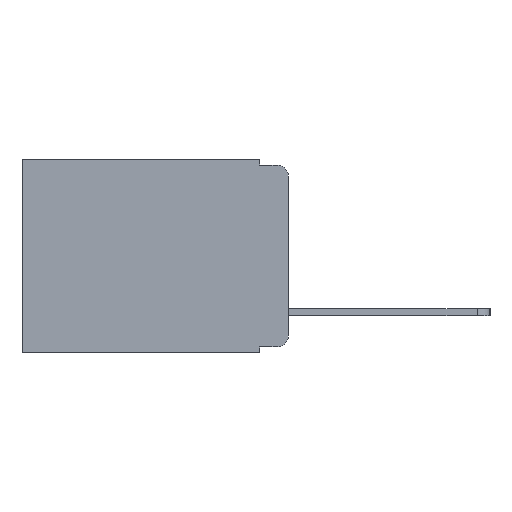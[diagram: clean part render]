
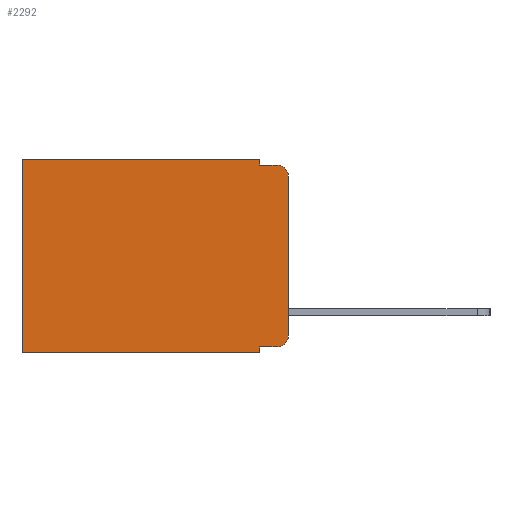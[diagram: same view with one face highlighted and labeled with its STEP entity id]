
A CAD part, left-side view. The second image highlights one B-rep face of the part: STEP entity #2292.
In plain terms, the highlighted planar face has unit normal (-1, 0, 0).
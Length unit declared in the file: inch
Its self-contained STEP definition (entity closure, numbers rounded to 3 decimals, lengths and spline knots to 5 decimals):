
#29 = VECTOR ( 'NONE', #2851, 39.37008 ) ;
#91 = CARTESIAN_POINT ( 'NONE',  ( 0.298, 0., -0.03 ) ) ;
#200 = VERTEX_POINT ( 'NONE', #11408 ) ;
#217 = VERTEX_POINT ( 'NONE', #91 ) ;
#716 = ORIENTED_EDGE ( 'NONE', *, *, #11020, .T. ) ;
#831 = VERTEX_POINT ( 'NONE', #9198 ) ;
#1003 = CARTESIAN_POINT ( 'NONE',  ( 0.298, 0.02, -0.313 ) ) ;
#1199 = DIRECTION ( 'NONE',  ( 0., 0., -1. ) ) ;
#1914 = LINE ( 'NONE', #3149, #4839 ) ;
#2048 = CIRCLE ( 'NONE', #6369, 0.02 ) ;
#2124 = ORIENTED_EDGE ( 'NONE', *, *, #7996, .F. ) ;
#2213 = VERTEX_POINT ( 'NONE', #3169 ) ;
#2292 = ADVANCED_FACE ( 'NONE', ( #11726 ), #14137, .F. ) ;
#2393 = CARTESIAN_POINT ( 'NONE',  ( 0.298, 0.473, 0. ) ) ;
#2446 = AXIS2_PLACEMENT_3D ( 'NONE', #1003, #14285, #14223 ) ;
#2461 = CARTESIAN_POINT ( 'NONE',  ( 0.298, 0.051, 0. ) ) ;
#2665 = CARTESIAN_POINT ( 'NONE',  ( 0.298, 0.051, 0. ) ) ;
#2746 = DIRECTION ( 'NONE',  ( 0., 1., 0. ) ) ;
#2770 = VECTOR ( 'NONE', #6279, 39.37008 ) ;
#2771 = CARTESIAN_POINT ( 'NONE',  ( 0.298, 0.02, -0.01 ) ) ;
#2830 = EDGE_CURVE ( 'NONE', #13042, #7911, #5754, .T. ) ;
#2851 = DIRECTION ( 'NONE',  ( 0., -1., 0. ) ) ;
#2897 = EDGE_CURVE ( 'NONE', #200, #831, #11869, .T. ) ;
#2970 = EDGE_CURVE ( 'NONE', #7788, #13042, #1914, .T. ) ;
#3143 = VECTOR ( 'NONE', #9335, 39.37008 ) ;
#3149 = CARTESIAN_POINT ( 'NONE',  ( 0.298, 0.051, 0. ) ) ;
#3169 = CARTESIAN_POINT ( 'NONE',  ( 0.298, 0.473, 0. ) ) ;
#4089 = EDGE_LOOP ( 'NONE', ( #9327, #6643, #14251, #2124, #9512, #716, #8259, #5156, #11557, #9687 ) ) ;
#4388 = EDGE_CURVE ( 'NONE', #10369, #2213, #6398, .T. ) ;
#4839 = VECTOR ( 'NONE', #10660, 39.37008 ) ;
#4972 = CARTESIAN_POINT ( 'NONE',  ( 0.298, 0.473, -0.343 ) ) ;
#5156 = ORIENTED_EDGE ( 'NONE', *, *, #2970, .F. ) ;
#5302 = EDGE_CURVE ( 'NONE', #217, #831, #13013, .T. ) ;
#5439 = CARTESIAN_POINT ( 'NONE',  ( 0.298, 0.051, -0.01 ) ) ;
#5705 = EDGE_CURVE ( 'NONE', #9955, #10579, #6214, .T. ) ;
#5754 = LINE ( 'NONE', #8586, #7348 ) ;
#5957 = LINE ( 'NONE', #2665, #2770 ) ;
#6214 = LINE ( 'NONE', #12013, #29 ) ;
#6279 = DIRECTION ( 'NONE',  ( 0., 0., -1. ) ) ;
#6308 = LINE ( 'NONE', #12542, #3143 ) ;
#6369 = AXIS2_PLACEMENT_3D ( 'NONE', #14941, #8399, #1199 ) ;
#6398 = LINE ( 'NONE', #11921, #9456 ) ;
#6643 = ORIENTED_EDGE ( 'NONE', *, *, #14168, .T. ) ;
#7348 = VECTOR ( 'NONE', #8561, 39.37008 ) ;
#7788 = VERTEX_POINT ( 'NONE', #14803 ) ;
#7911 = VERTEX_POINT ( 'NONE', #4972 ) ;
#7996 = EDGE_CURVE ( 'NONE', #10369, #9955, #5957, .T. ) ;
#8259 = ORIENTED_EDGE ( 'NONE', *, *, #2830, .F. ) ;
#8399 = DIRECTION ( 'NONE',  ( -1., 0., 0. ) ) ;
#8487 = EDGE_CURVE ( 'NONE', #7788, #200, #6308, .T. ) ;
#8561 = DIRECTION ( 'NONE',  ( 0., 1., 0. ) ) ;
#8586 = CARTESIAN_POINT ( 'NONE',  ( 0.298, 0., -0.343 ) ) ;
#9198 = CARTESIAN_POINT ( 'NONE',  ( 0.298, 0., -0.313 ) ) ;
#9327 = ORIENTED_EDGE ( 'NONE', *, *, #5302, .F. ) ;
#9335 = DIRECTION ( 'NONE',  ( 0., -1., 0. ) ) ;
#9456 = VECTOR ( 'NONE', #2746, 39.37008 ) ;
#9512 = ORIENTED_EDGE ( 'NONE', *, *, #4388, .T. ) ;
#9687 = ORIENTED_EDGE ( 'NONE', *, *, #2897, .T. ) ;
#9899 = AXIS2_PLACEMENT_3D ( 'NONE', #12950, #13815, #13828 ) ;
#9955 = VERTEX_POINT ( 'NONE', #5439 ) ;
#10074 = CARTESIAN_POINT ( 'NONE',  ( 0.298, 0.051, -0.343 ) ) ;
#10192 = VECTOR ( 'NONE', #14170, 39.37008 ) ;
#10369 = VERTEX_POINT ( 'NONE', #2461 ) ;
#10554 = DIRECTION ( 'NONE',  ( 0., 0., -1. ) ) ;
#10579 = VERTEX_POINT ( 'NONE', #2771 ) ;
#10660 = DIRECTION ( 'NONE',  ( 0., 0., -1. ) ) ;
#10920 = CARTESIAN_POINT ( 'NONE',  ( 0.298, 0., 0. ) ) ;
#11020 = EDGE_CURVE ( 'NONE', #2213, #7911, #13910, .T. ) ;
#11042 = VECTOR ( 'NONE', #10554, 39.37008 ) ;
#11408 = CARTESIAN_POINT ( 'NONE',  ( 0.298, 0.02, -0.333 ) ) ;
#11557 = ORIENTED_EDGE ( 'NONE', *, *, #8487, .T. ) ;
#11726 = FACE_OUTER_BOUND ( 'NONE', #4089, .T. ) ;
#11869 = CIRCLE ( 'NONE', #2446, 0.02 ) ;
#11921 = CARTESIAN_POINT ( 'NONE',  ( 0.298, 0., 0. ) ) ;
#12013 = CARTESIAN_POINT ( 'NONE',  ( 0.298, 0.051, -0.01 ) ) ;
#12542 = CARTESIAN_POINT ( 'NONE',  ( 0.298, 0.051, -0.333 ) ) ;
#12950 = CARTESIAN_POINT ( 'NONE',  ( 0.298, 0., 0. ) ) ;
#13013 = LINE ( 'NONE', #10920, #10192 ) ;
#13042 = VERTEX_POINT ( 'NONE', #10074 ) ;
#13815 = DIRECTION ( 'NONE',  ( 1., 0., 0. ) ) ;
#13828 = DIRECTION ( 'NONE',  ( 0., 0., -1. ) ) ;
#13910 = LINE ( 'NONE', #2393, #11042 ) ;
#14137 = PLANE ( 'NONE',  #9899 ) ;
#14168 = EDGE_CURVE ( 'NONE', #217, #10579, #2048, .T. ) ;
#14170 = DIRECTION ( 'NONE',  ( 0., 0., -1. ) ) ;
#14223 = DIRECTION ( 'NONE',  ( 0., 0., -1. ) ) ;
#14251 = ORIENTED_EDGE ( 'NONE', *, *, #5705, .F. ) ;
#14285 = DIRECTION ( 'NONE',  ( -1., 0., 0. ) ) ;
#14803 = CARTESIAN_POINT ( 'NONE',  ( 0.298, 0.051, -0.333 ) ) ;
#14941 = CARTESIAN_POINT ( 'NONE',  ( 0.298, 0.02, -0.03 ) ) ;
